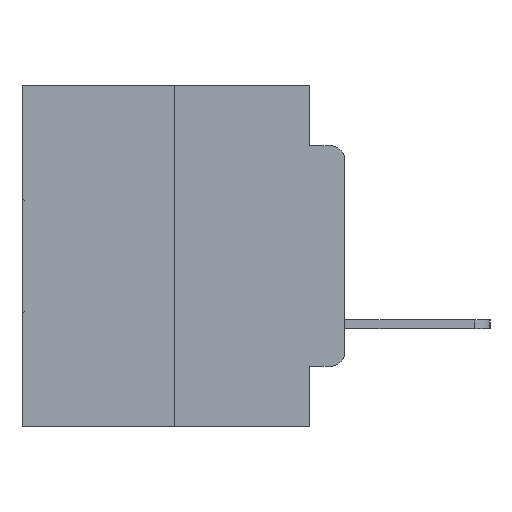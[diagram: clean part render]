
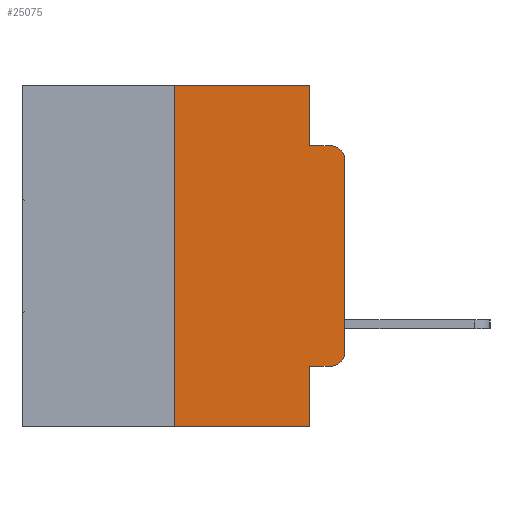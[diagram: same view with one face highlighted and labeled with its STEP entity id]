
A CAD part, left-side view. The second image highlights one B-rep face of the part: STEP entity #25075.
In plain terms, the highlighted planar face has unit normal (-1, 0, 0).
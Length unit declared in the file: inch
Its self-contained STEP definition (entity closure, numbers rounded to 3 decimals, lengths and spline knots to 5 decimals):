
#124 = DIRECTION ( 'NONE',  ( 0., -1., 0. ) ) ;
#128 = EDGE_CURVE ( 'NONE', #25180, #24576, #6207, .T. ) ;
#545 = CARTESIAN_POINT ( 'NONE',  ( 0., 0.051, -0.4115 ) ) ;
#911 = DIRECTION ( 'NONE',  ( 0., 0., -1. ) ) ;
#1965 = DIRECTION ( 'NONE',  ( 0., 0., 1. ) ) ;
#2079 = EDGE_CURVE ( 'NONE', #10433, #2688, #22841, .T. ) ;
#2299 = ORIENTED_EDGE ( 'NONE', *, *, #9301, .F. ) ;
#2688 = VERTEX_POINT ( 'NONE', #5238 ) ;
#3511 = DIRECTION ( 'NONE',  ( 0., 0., -1. ) ) ;
#3951 = PLANE ( 'NONE',  #10349 ) ;
#4166 = EDGE_CURVE ( 'NONE', #8849, #12364, #11329, .T. ) ;
#4750 = LINE ( 'NONE', #7853, #27001 ) ;
#4943 = LINE ( 'NONE', #11582, #11448 ) ;
#4973 = DIRECTION ( 'NONE',  ( 0., -1., 0. ) ) ;
#5238 = CARTESIAN_POINT ( 'NONE',  ( 0., 0.051, -0.0885 ) ) ;
#5419 = LINE ( 'NONE', #20638, #16998 ) ;
#5487 = VERTEX_POINT ( 'NONE', #25584 ) ;
#6177 = CARTESIAN_POINT ( 'NONE',  ( 0., 0.473, 0. ) ) ;
#6207 = LINE ( 'NONE', #545, #22060 ) ;
#6783 = VECTOR ( 'NONE', #18239, 39.37008 ) ;
#7408 = EDGE_CURVE ( 'NONE', #21104, #17728, #19759, .T. ) ;
#7476 = LINE ( 'NONE', #26697, #6783 ) ;
#7526 = ORIENTED_EDGE ( 'NONE', *, *, #128, .T. ) ;
#7596 = EDGE_LOOP ( 'NONE', ( #18001, #27322, #21236, #9923, #13009, #21146, #8226, #2299, #7526, #16380 ) ) ;
#7853 = CARTESIAN_POINT ( 'NONE',  ( 0., 0.051, 0. ) ) ;
#7880 = CARTESIAN_POINT ( 'NONE',  ( 0., 0., -0.3915 ) ) ;
#8226 = ORIENTED_EDGE ( 'NONE', *, *, #7408, .T. ) ;
#8370 = DIRECTION ( 'NONE',  ( 1., 0., 0. ) ) ;
#8849 = VERTEX_POINT ( 'NONE', #15015 ) ;
#9301 = EDGE_CURVE ( 'NONE', #25180, #17728, #4750, .T. ) ;
#9480 = EDGE_CURVE ( 'NONE', #22098, #8849, #12286, .T. ) ;
#9534 = CARTESIAN_POINT ( 'NONE',  ( 0., 0.25, -0.5 ) ) ;
#9923 = ORIENTED_EDGE ( 'NONE', *, *, #2079, .F. ) ;
#10349 = AXIS2_PLACEMENT_3D ( 'NONE', #6177, #8370, #23451 ) ;
#10433 = VERTEX_POINT ( 'NONE', #13984 ) ;
#11329 = CIRCLE ( 'NONE', #18780, 0.02 ) ;
#11448 = VECTOR ( 'NONE', #4973, 39.37008 ) ;
#11582 = CARTESIAN_POINT ( 'NONE',  ( 0., 0.051, -0.0885 ) ) ;
#12286 = LINE ( 'NONE', #27825, #16683 ) ;
#12364 = VERTEX_POINT ( 'NONE', #25143 ) ;
#12709 = DIRECTION ( 'NONE',  ( -1., 0., 0. ) ) ;
#13009 = ORIENTED_EDGE ( 'NONE', *, *, #17860, .F. ) ;
#13131 = CARTESIAN_POINT ( 'NONE',  ( 0., 0.02, -0.3915 ) ) ;
#13984 = CARTESIAN_POINT ( 'NONE',  ( 0., 0.051, 0. ) ) ;
#15015 = CARTESIAN_POINT ( 'NONE',  ( 0., 0., -0.1085 ) ) ;
#15146 = CARTESIAN_POINT ( 'NONE',  ( 0., 0.02, -0.4115 ) ) ;
#15293 = DIRECTION ( 'NONE',  ( 0., 0., -1. ) ) ;
#15393 = DIRECTION ( 'NONE',  ( 0., -1., 0. ) ) ;
#16380 = ORIENTED_EDGE ( 'NONE', *, *, #25182, .T. ) ;
#16683 = VECTOR ( 'NONE', #1965, 39.37008 ) ;
#16998 = VECTOR ( 'NONE', #22816, 39.37008 ) ;
#17166 = VECTOR ( 'NONE', #911, 39.37008 ) ;
#17728 = VERTEX_POINT ( 'NONE', #22246 ) ;
#17779 = EDGE_CURVE ( 'NONE', #21104, #5487, #7476, .T. ) ;
#17860 = EDGE_CURVE ( 'NONE', #5487, #10433, #5419, .T. ) ;
#18001 = ORIENTED_EDGE ( 'NONE', *, *, #9480, .T. ) ;
#18239 = DIRECTION ( 'NONE',  ( 0., 0., 1. ) ) ;
#18264 = CARTESIAN_POINT ( 'NONE',  ( 0., 0.051, 0. ) ) ;
#18780 = AXIS2_PLACEMENT_3D ( 'NONE', #25541, #12709, #27654 ) ;
#19759 = LINE ( 'NONE', #26025, #26773 ) ;
#20423 = AXIS2_PLACEMENT_3D ( 'NONE', #13131, #28039, #15293 ) ;
#20638 = CARTESIAN_POINT ( 'NONE',  ( 0., 0.473, 0. ) ) ;
#21104 = VERTEX_POINT ( 'NONE', #9534 ) ;
#21146 = ORIENTED_EDGE ( 'NONE', *, *, #17779, .F. ) ;
#21155 = CIRCLE ( 'NONE', #20423, 0.02 ) ;
#21236 = ORIENTED_EDGE ( 'NONE', *, *, #21678, .F. ) ;
#21633 = CARTESIAN_POINT ( 'NONE',  ( 0., 0.051, -0.4115 ) ) ;
#21678 = EDGE_CURVE ( 'NONE', #2688, #12364, #4943, .T. ) ;
#22060 = VECTOR ( 'NONE', #124, 39.37008 ) ;
#22098 = VERTEX_POINT ( 'NONE', #7880 ) ;
#22246 = CARTESIAN_POINT ( 'NONE',  ( 0., 0.051, -0.5 ) ) ;
#22816 = DIRECTION ( 'NONE',  ( 0., -1., 0. ) ) ;
#22841 = LINE ( 'NONE', #18264, #17166 ) ;
#23451 = DIRECTION ( 'NONE',  ( 0., 0., -1. ) ) ;
#24516 = FACE_OUTER_BOUND ( 'NONE', #7596, .T. ) ;
#24576 = VERTEX_POINT ( 'NONE', #15146 ) ;
#25075 = ADVANCED_FACE ( 'NONE', ( #24516 ), #3951, .F. ) ;
#25143 = CARTESIAN_POINT ( 'NONE',  ( 0., 0.02, -0.0885 ) ) ;
#25180 = VERTEX_POINT ( 'NONE', #21633 ) ;
#25182 = EDGE_CURVE ( 'NONE', #24576, #22098, #21155, .T. ) ;
#25541 = CARTESIAN_POINT ( 'NONE',  ( 0., 0.02, -0.1085 ) ) ;
#25584 = CARTESIAN_POINT ( 'NONE',  ( 0., 0.25, 0. ) ) ;
#26025 = CARTESIAN_POINT ( 'NONE',  ( 0., 0.473, -0.5 ) ) ;
#26697 = CARTESIAN_POINT ( 'NONE',  ( 0., 0.25, 0. ) ) ;
#26773 = VECTOR ( 'NONE', #15393, 39.37008 ) ;
#27001 = VECTOR ( 'NONE', #3511, 39.37008 ) ;
#27322 = ORIENTED_EDGE ( 'NONE', *, *, #4166, .T. ) ;
#27654 = DIRECTION ( 'NONE',  ( 0., 0., -1. ) ) ;
#27825 = CARTESIAN_POINT ( 'NONE',  ( 0., 0., 0. ) ) ;
#28039 = DIRECTION ( 'NONE',  ( -1., 0., 0. ) ) ;
